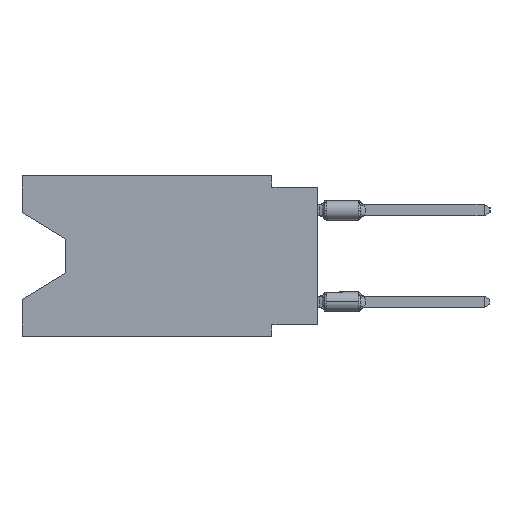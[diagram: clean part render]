
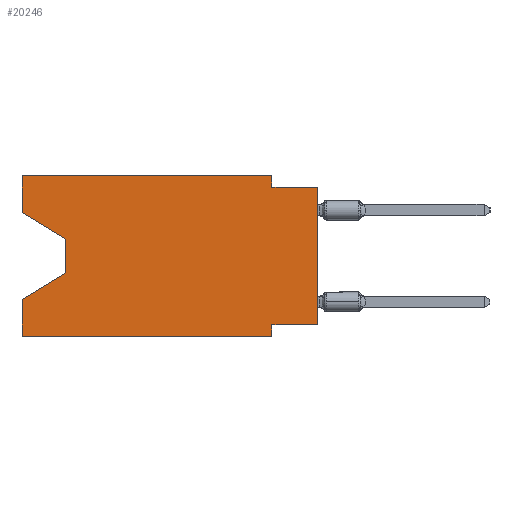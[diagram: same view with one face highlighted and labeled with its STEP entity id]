
A CAD part, left-side view. The second image highlights one B-rep face of the part: STEP entity #20246.
In plain terms, the highlighted planar face has unit normal (-1, 0, 0).
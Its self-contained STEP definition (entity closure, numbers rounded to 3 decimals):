
#637 = ORIENTED_EDGE ( 'NONE', *, *, #44693, .F. ) ;
#1548 = DIRECTION ( 'NONE',  ( 0., -0.855, -0.519 ) ) ;
#3003 = VERTEX_POINT ( 'NONE', #8368 ) ;
#3707 = VECTOR ( 'NONE', #11857, 1000. ) ;
#3925 = DIRECTION ( 'NONE',  ( 0., 1., 0. ) ) ;
#4057 = DIRECTION ( 'NONE',  ( 0., 0., 1. ) ) ;
#4973 = LINE ( 'NONE', #18911, #32657 ) ;
#5551 = EDGE_CURVE ( 'NONE', #32247, #34372, #12481, .T. ) ;
#6622 = VERTEX_POINT ( 'NONE', #41800 ) ;
#6732 = EDGE_CURVE ( 'NONE', #3003, #34039, #8161, .T. ) ;
#7283 = DIRECTION ( 'NONE',  ( 0., -1., 0. ) ) ;
#7430 = VERTEX_POINT ( 'NONE', #42863 ) ;
#7752 = DIRECTION ( 'NONE',  ( 0., 0., 1. ) ) ;
#8161 = LINE ( 'NONE', #24626, #12179 ) ;
#8219 = VERTEX_POINT ( 'NONE', #15148 ) ;
#8368 = CARTESIAN_POINT ( 'NONE',  ( 0., 16.383, -2.038 ) ) ;
#8863 = VECTOR ( 'NONE', #3925, 1000. ) ;
#9093 = ORIENTED_EDGE ( 'NONE', *, *, #18528, .T. ) ;
#9870 = VECTOR ( 'NONE', #7752, 1000. ) ;
#10362 = FACE_OUTER_BOUND ( 'NONE', #11866, .T. ) ;
#10814 = DIRECTION ( 'NONE',  ( 1., 0., 0. ) ) ;
#11198 = EDGE_CURVE ( 'NONE', #41825, #32247, #27498, .T. ) ;
#11564 = DIRECTION ( 'NONE',  ( 0., -1., 0. ) ) ;
#11857 = DIRECTION ( 'NONE',  ( 0., -1., 0. ) ) ;
#11866 = EDGE_LOOP ( 'NONE', ( #12492, #35456, #34890, #22207, #16294, #23432, #40894, #9093, #22949, #637, #16520, #33640 ) ) ;
#12179 = VECTOR ( 'NONE', #4057, 1000. ) ;
#12421 = VECTOR ( 'NONE', #17101, 1000. ) ;
#12481 = LINE ( 'NONE', #22974, #19429 ) ;
#12492 = ORIENTED_EDGE ( 'NONE', *, *, #13090, .T. ) ;
#12921 = CARTESIAN_POINT ( 'NONE',  ( 0., 2.54, -0.635 ) ) ;
#13090 = EDGE_CURVE ( 'NONE', #3003, #7430, #4973, .T. ) ;
#13905 = LINE ( 'NONE', #24638, #12421 ) ;
#14053 = CARTESIAN_POINT ( 'NONE',  ( 0., 0., -8.255 ) ) ;
#14182 = VECTOR ( 'NONE', #29933, 1000. ) ;
#15049 = CARTESIAN_POINT ( 'NONE',  ( 0., 16.383, 0. ) ) ;
#15148 = CARTESIAN_POINT ( 'NONE',  ( 0., 16.383, -6.852 ) ) ;
#15221 = CARTESIAN_POINT ( 'NONE',  ( 0., 0., -0.635 ) ) ;
#15290 = CARTESIAN_POINT ( 'NONE',  ( 0., 16.383, 0. ) ) ;
#15626 = LINE ( 'NONE', #23373, #21148 ) ;
#15666 = DIRECTION ( 'NONE',  ( 0., 0., 1. ) ) ;
#16010 = EDGE_CURVE ( 'NONE', #7430, #35112, #13905, .T. ) ;
#16112 = LINE ( 'NONE', #29203, #30102 ) ;
#16294 = ORIENTED_EDGE ( 'NONE', *, *, #17200, .T. ) ;
#16520 = ORIENTED_EDGE ( 'NONE', *, *, #29988, .F. ) ;
#16647 = VERTEX_POINT ( 'NONE', #43338 ) ;
#17060 = CARTESIAN_POINT ( 'NONE',  ( 0., 2.54, -8.89 ) ) ;
#17101 = DIRECTION ( 'NONE',  ( 0., 0., -1. ) ) ;
#17200 = EDGE_CURVE ( 'NONE', #6622, #34372, #24647, .T. ) ;
#18528 = EDGE_CURVE ( 'NONE', #41825, #16647, #16112, .T. ) ;
#18737 = VERTEX_POINT ( 'NONE', #12921 ) ;
#18911 = CARTESIAN_POINT ( 'NONE',  ( 0., 16.383, -2.038 ) ) ;
#19285 = EDGE_CURVE ( 'NONE', #18737, #16647, #42914, .T. ) ;
#19429 = VECTOR ( 'NONE', #43606, 1000. ) ;
#20246 = ADVANCED_FACE ( 'NONE', ( #10362 ), #28205, .F. ) ;
#20786 = CARTESIAN_POINT ( 'NONE',  ( 0., 13.97, -5.385 ) ) ;
#21148 = VECTOR ( 'NONE', #36674, 1000. ) ;
#21233 = CARTESIAN_POINT ( 'NONE',  ( 0., 16.383, 0. ) ) ;
#22207 = ORIENTED_EDGE ( 'NONE', *, *, #37381, .F. ) ;
#22879 = AXIS2_PLACEMENT_3D ( 'NONE', #31636, #10814, #24288 ) ;
#22949 = ORIENTED_EDGE ( 'NONE', *, *, #19285, .F. ) ;
#22974 = CARTESIAN_POINT ( 'NONE',  ( 0., 2.54, -8.89 ) ) ;
#23373 = CARTESIAN_POINT ( 'NONE',  ( 0., 2.54, 0. ) ) ;
#23432 = ORIENTED_EDGE ( 'NONE', *, *, #5551, .F. ) ;
#24288 = DIRECTION ( 'NONE',  ( 0., 0., -1. ) ) ;
#24626 = CARTESIAN_POINT ( 'NONE',  ( 0., 16.383, 0. ) ) ;
#24638 = CARTESIAN_POINT ( 'NONE',  ( 0., 13.97, -3.505 ) ) ;
#24647 = LINE ( 'NONE', #45058, #38811 ) ;
#24932 = CARTESIAN_POINT ( 'NONE',  ( 0., 0., -8.255 ) ) ;
#27498 = LINE ( 'NONE', #24932, #8863 ) ;
#27996 = CARTESIAN_POINT ( 'NONE',  ( 0., 2.54, 0. ) ) ;
#28205 = PLANE ( 'NONE',  #22879 ) ;
#28241 = EDGE_CURVE ( 'NONE', #35112, #8219, #34475, .T. ) ;
#29203 = CARTESIAN_POINT ( 'NONE',  ( 0., 0., 0. ) ) ;
#29933 = DIRECTION ( 'NONE',  ( 0., 0.855, -0.519 ) ) ;
#29988 = EDGE_CURVE ( 'NONE', #34039, #32077, #42986, .T. ) ;
#30102 = VECTOR ( 'NONE', #15666, 1000. ) ;
#31636 = CARTESIAN_POINT ( 'NONE',  ( 0., 16.383, 0. ) ) ;
#32077 = VERTEX_POINT ( 'NONE', #27996 ) ;
#32247 = VERTEX_POINT ( 'NONE', #43100 ) ;
#32657 = VECTOR ( 'NONE', #1548, 1000. ) ;
#33640 = ORIENTED_EDGE ( 'NONE', *, *, #6732, .F. ) ;
#34039 = VERTEX_POINT ( 'NONE', #15049 ) ;
#34372 = VERTEX_POINT ( 'NONE', #17060 ) ;
#34475 = LINE ( 'NONE', #43886, #14182 ) ;
#34890 = ORIENTED_EDGE ( 'NONE', *, *, #28241, .T. ) ;
#35112 = VERTEX_POINT ( 'NONE', #20786 ) ;
#35456 = ORIENTED_EDGE ( 'NONE', *, *, #16010, .T. ) ;
#36674 = DIRECTION ( 'NONE',  ( 0., 0., -1. ) ) ;
#37381 = EDGE_CURVE ( 'NONE', #6622, #8219, #39087, .T. ) ;
#38811 = VECTOR ( 'NONE', #7283, 1000. ) ;
#39087 = LINE ( 'NONE', #21233, #9870 ) ;
#40894 = ORIENTED_EDGE ( 'NONE', *, *, #11198, .F. ) ;
#41800 = CARTESIAN_POINT ( 'NONE',  ( 0., 16.383, -8.89 ) ) ;
#41825 = VERTEX_POINT ( 'NONE', #14053 ) ;
#42567 = VECTOR ( 'NONE', #11564, 1000. ) ;
#42863 = CARTESIAN_POINT ( 'NONE',  ( 0., 13.97, -3.505 ) ) ;
#42914 = LINE ( 'NONE', #15221, #42567 ) ;
#42986 = LINE ( 'NONE', #15290, #3707 ) ;
#43100 = CARTESIAN_POINT ( 'NONE',  ( 0., 2.54, -8.255 ) ) ;
#43338 = CARTESIAN_POINT ( 'NONE',  ( 0., 0., -0.635 ) ) ;
#43606 = DIRECTION ( 'NONE',  ( 0., 0., -1. ) ) ;
#43886 = CARTESIAN_POINT ( 'NONE',  ( 0., 13.97, -5.385 ) ) ;
#44693 = EDGE_CURVE ( 'NONE', #32077, #18737, #15626, .T. ) ;
#45058 = CARTESIAN_POINT ( 'NONE',  ( 0., 16.383, -8.89 ) ) ;
